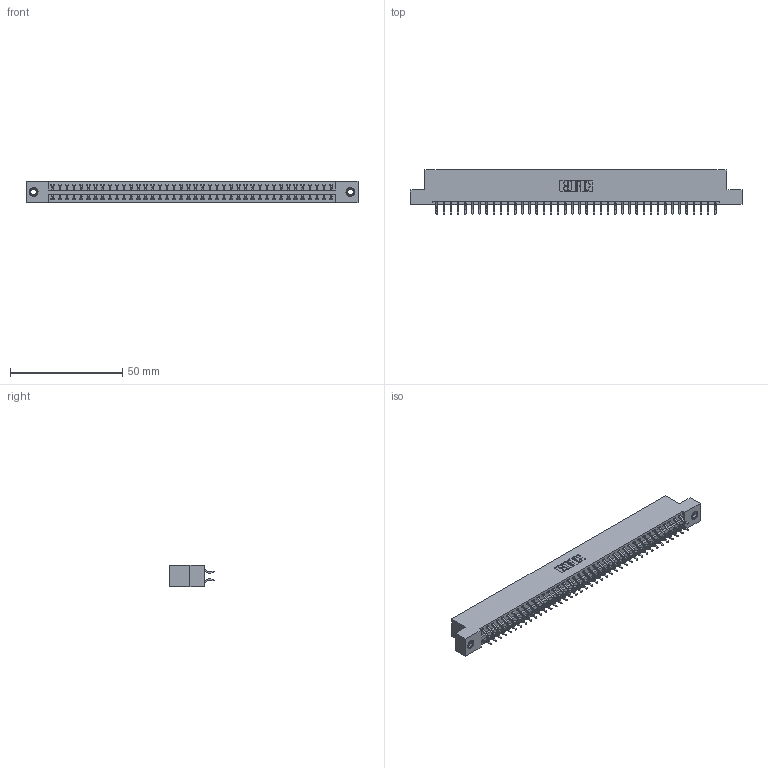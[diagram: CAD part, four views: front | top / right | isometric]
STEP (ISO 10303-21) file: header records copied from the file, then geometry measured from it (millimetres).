
FILE_DESCRIPTION (( 'STEP AP203' ), '1' );
FILE_NAME ('396-080-556-207.STEP', '2018-09-09T21:22:56', ( '' ), ( '' ), 'SwSTEP 2.0', 'SolidWorks 2016', '' );
FILE_SCHEMA (( 'CONFIG_CONTROL_DESIGN' ));
Length unit declared in the file: inch
Products named in the file (4): 346 Part_Flush Mounting Lugs - 0.156 Dia-TI; 345-292-001_556 Tail; 345-250-001_345-250-005-103; 396-080-556-207
Assembly tree (83 placements, depth 2):
  396-080-556-207
    346 Part_Flush Mounting Lugs - 0.156 Dia-TI
    345-292-001_556 Tail  x80
    345-250-001_345-250-005-103  x2
Bounding box: 147.57 x 19.57 x 9.4 mm (x, y, z)
Volume: 14358.1 mm3; surface area: 19664.1 mm2
Topology: 83 solids, 83 shells, 4822 faces, 14305 edges, 9422 vertices
Faces by surface type: plane 3228, cylinder 1578, cone 12, torus 4
Entity records: 27780 total; most frequent: CARTESIAN_POINT 4579, ORIENTED_EDGE 4494, DIRECTION 4101, EDGE_CURVE 2247, VECTOR 1927, LINE 1927, VERTEX_POINT 1492, AXIS2_PLACEMENT_3D 1087
